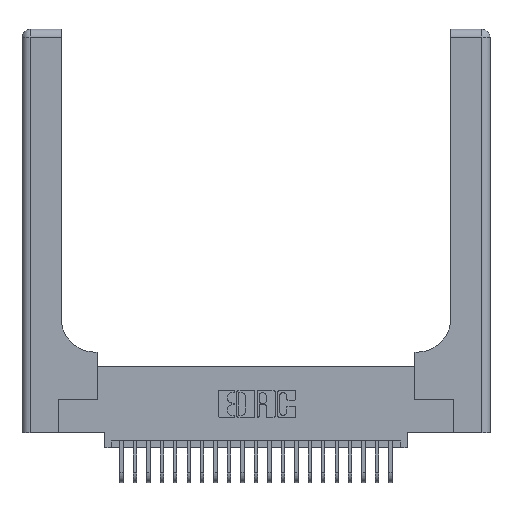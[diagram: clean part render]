
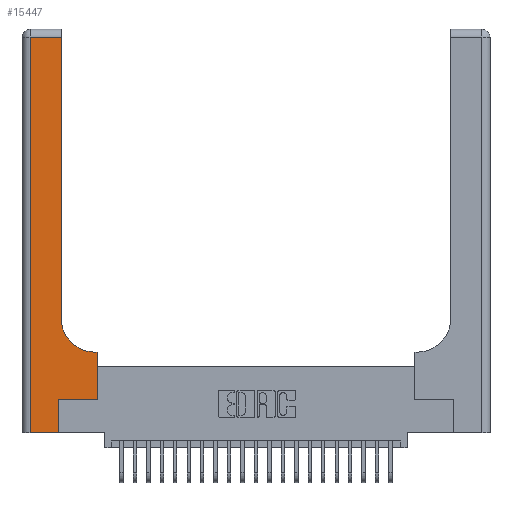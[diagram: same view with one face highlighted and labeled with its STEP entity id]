
A CAD part, top view. The second image highlights one B-rep face of the part: STEP entity #15447.
In plain terms, the highlighted planar face has unit normal (0, 0, 1).
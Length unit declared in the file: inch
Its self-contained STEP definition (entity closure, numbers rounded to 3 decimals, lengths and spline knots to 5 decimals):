
#375 = CARTESIAN_POINT ( 'NONE',  ( 0.2915, 2.94, 0.37 ) ) ;
#709 = CARTESIAN_POINT ( 'NONE',  ( 0.5585, 0.25, 0.37 ) ) ;
#740 = CARTESIAN_POINT ( 'NONE',  ( 0., 3., 0.37 ) ) ;
#898 = ORIENTED_EDGE ( 'NONE', *, *, #15037, .T. ) ;
#1356 = ORIENTED_EDGE ( 'NONE', *, *, #1908, .T. ) ;
#1787 = CIRCLE ( 'NONE', #14109, 0.25 ) ;
#1908 = EDGE_CURVE ( 'NONE', #4787, #25434, #13744, .T. ) ;
#2763 = DIRECTION ( 'NONE',  ( 0., 1., 0. ) ) ;
#2800 = DIRECTION ( 'NONE',  ( -1., 0., 0. ) ) ;
#2922 = VECTOR ( 'NONE', #20824, 39.37008 ) ;
#3548 = CARTESIAN_POINT ( 'NONE',  ( 0.06, 0., 0.37 ) ) ;
#3889 = VECTOR ( 'NONE', #2763, 39.37008 ) ;
#4206 = EDGE_CURVE ( 'NONE', #13684, #4787, #17414, .T. ) ;
#4787 = VERTEX_POINT ( 'NONE', #3548 ) ;
#5455 = FACE_OUTER_BOUND ( 'NONE', #18526, .T. ) ;
#5659 = CARTESIAN_POINT ( 'NONE',  ( 0.2915, 3., 0.37 ) ) ;
#5774 = EDGE_CURVE ( 'NONE', #20712, #9934, #20149, .T. ) ;
#6145 = LINE ( 'NONE', #5659, #15718 ) ;
#6214 = DIRECTION ( 'NONE',  ( 0., -1., 0. ) ) ;
#6582 = CARTESIAN_POINT ( 'NONE',  ( 0.5415, 0.85, 0.37 ) ) ;
#6669 = CARTESIAN_POINT ( 'NONE',  ( 0.269, 0.25, 0.37 ) ) ;
#6892 = ORIENTED_EDGE ( 'NONE', *, *, #9287, .T. ) ;
#6914 = ORIENTED_EDGE ( 'NONE', *, *, #22607, .T. ) ;
#7485 = DIRECTION ( 'NONE',  ( -1., 0., 0. ) ) ;
#7530 = VECTOR ( 'NONE', #24712, 39.37008 ) ;
#7556 = ORIENTED_EDGE ( 'NONE', *, *, #19779, .T. ) ;
#7967 = VERTEX_POINT ( 'NONE', #17620 ) ;
#8411 = AXIS2_PLACEMENT_3D ( 'NONE', #740, #15119, #2800 ) ;
#8667 = DIRECTION ( 'NONE',  ( 1., 0., 0. ) ) ;
#8999 = CARTESIAN_POINT ( 'NONE',  ( 0.5585, 0.6, 0.37 ) ) ;
#9287 = EDGE_CURVE ( 'NONE', #7967, #20712, #24531, .T. ) ;
#9934 = VERTEX_POINT ( 'NONE', #8999 ) ;
#10025 = CARTESIAN_POINT ( 'NONE',  ( 0.269, 0., 0.37 ) ) ;
#11902 = ORIENTED_EDGE ( 'NONE', *, *, #4206, .T. ) ;
#11918 = VECTOR ( 'NONE', #24033, 39.37008 ) ;
#12471 = CARTESIAN_POINT ( 'NONE',  ( 0.06, 2.94, 0.37 ) ) ;
#13011 = PLANE ( 'NONE',  #8411 ) ;
#13571 = LINE ( 'NONE', #22699, #7530 ) ;
#13684 = VERTEX_POINT ( 'NONE', #12471 ) ;
#13744 = LINE ( 'NONE', #24134, #23790 ) ;
#14109 = AXIS2_PLACEMENT_3D ( 'NONE', #6582, #20740, #8667 ) ;
#14195 = VERTEX_POINT ( 'NONE', #24111 ) ;
#15037 = EDGE_CURVE ( 'NONE', #14195, #23142, #6145, .T. ) ;
#15119 = DIRECTION ( 'NONE',  ( 0., 0., -1. ) ) ;
#15447 = ADVANCED_FACE ( 'NONE', ( #5455 ), #13011, .F. ) ;
#15718 = VECTOR ( 'NONE', #23901, 39.37008 ) ;
#15730 = EDGE_CURVE ( 'NONE', #25434, #7967, #20085, .T. ) ;
#16602 = ORIENTED_EDGE ( 'NONE', *, *, #15730, .T. ) ;
#16765 = VECTOR ( 'NONE', #6214, 39.37008 ) ;
#17354 = EDGE_CURVE ( 'NONE', #23142, #13684, #22185, .T. ) ;
#17414 = LINE ( 'NONE', #22415, #16765 ) ;
#17620 = CARTESIAN_POINT ( 'NONE',  ( 0.269, 0.25, 0.37 ) ) ;
#17791 = ORIENTED_EDGE ( 'NONE', *, *, #5774, .T. ) ;
#18186 = CARTESIAN_POINT ( 'NONE',  ( 0.5415, 0.6, 0.37 ) ) ;
#18511 = ORIENTED_EDGE ( 'NONE', *, *, #17354, .T. ) ;
#18526 = EDGE_LOOP ( 'NONE', ( #898, #18511, #11902, #1356, #16602, #6892, #17791, #7556, #6914 ) ) ;
#19594 = CARTESIAN_POINT ( 'NONE',  ( 0., 2.94, 0.37 ) ) ;
#19779 = EDGE_CURVE ( 'NONE', #9934, #26223, #13571, .T. ) ;
#20085 = LINE ( 'NONE', #10025, #11918 ) ;
#20149 = LINE ( 'NONE', #709, #3889 ) ;
#20712 = VERTEX_POINT ( 'NONE', #22411 ) ;
#20740 = DIRECTION ( 'NONE',  ( 0., 0., -1. ) ) ;
#20824 = DIRECTION ( 'NONE',  ( 1., 0., 0. ) ) ;
#21566 = VECTOR ( 'NONE', #7485, 39.37008 ) ;
#22185 = LINE ( 'NONE', #19594, #21566 ) ;
#22411 = CARTESIAN_POINT ( 'NONE',  ( 0.5585, 0.25, 0.37 ) ) ;
#22415 = CARTESIAN_POINT ( 'NONE',  ( 0.06, 3., 0.37 ) ) ;
#22607 = EDGE_CURVE ( 'NONE', #26223, #14195, #1787, .T. ) ;
#22699 = CARTESIAN_POINT ( 'NONE',  ( 0.2915, 0.6, 0.37 ) ) ;
#23142 = VERTEX_POINT ( 'NONE', #375 ) ;
#23790 = VECTOR ( 'NONE', #24102, 39.37008 ) ;
#23901 = DIRECTION ( 'NONE',  ( 0., 1., 0. ) ) ;
#24033 = DIRECTION ( 'NONE',  ( 0., 1., 0. ) ) ;
#24102 = DIRECTION ( 'NONE',  ( 1., 0., 0. ) ) ;
#24111 = CARTESIAN_POINT ( 'NONE',  ( 0.2915, 0.85, 0.37 ) ) ;
#24134 = CARTESIAN_POINT ( 'NONE',  ( 0., 0., 0.37 ) ) ;
#24531 = LINE ( 'NONE', #6669, #2922 ) ;
#24712 = DIRECTION ( 'NONE',  ( -1., 0., 0. ) ) ;
#25434 = VERTEX_POINT ( 'NONE', #25442 ) ;
#25442 = CARTESIAN_POINT ( 'NONE',  ( 0.269, 0., 0.37 ) ) ;
#26223 = VERTEX_POINT ( 'NONE', #18186 ) ;
